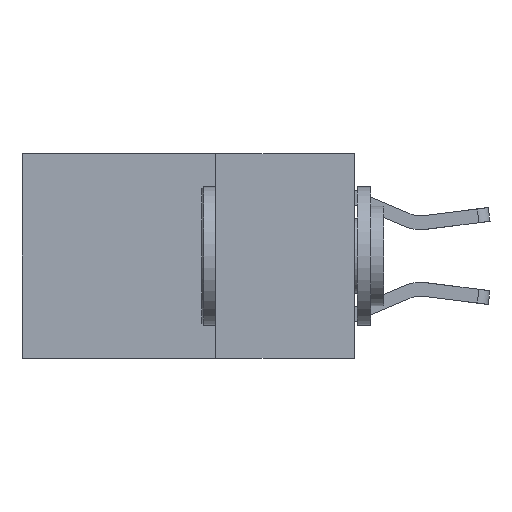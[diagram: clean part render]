
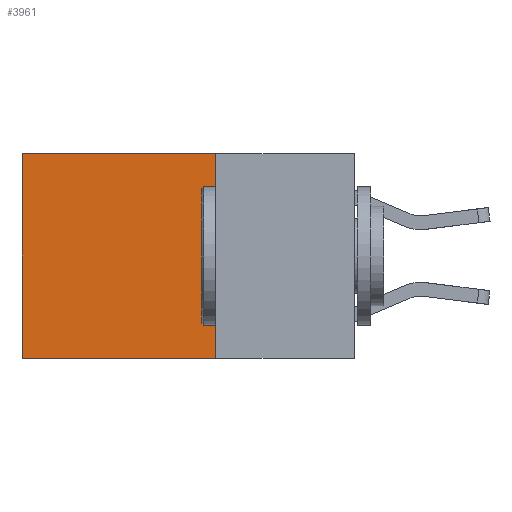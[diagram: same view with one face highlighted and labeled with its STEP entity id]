
A CAD part, left-side view. The second image highlights one B-rep face of the part: STEP entity #3961.
In plain terms, the highlighted planar face has unit normal (-1, 0, 0).
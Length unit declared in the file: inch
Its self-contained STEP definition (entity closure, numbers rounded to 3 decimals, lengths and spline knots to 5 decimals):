
#654 = DIRECTION ( 'NONE',  ( 1., 0., 0. ) ) ;
#752 = EDGE_LOOP ( 'NONE', ( #3261, #6210, #2704, #8444 ) ) ;
#809 = VECTOR ( 'NONE', #5398, 39.37008 ) ;
#868 = DIRECTION ( 'NONE',  ( 0., 0., -1. ) ) ;
#966 = CARTESIAN_POINT ( 'NONE',  ( 0.2625, 0.25, -0.37 ) ) ;
#1602 = LINE ( 'NONE', #6853, #809 ) ;
#1788 = CARTESIAN_POINT ( 'NONE',  ( 0.2625, 0.25, 0. ) ) ;
#2057 = VERTEX_POINT ( 'NONE', #5592 ) ;
#2075 = FACE_OUTER_BOUND ( 'NONE', #752, .T. ) ;
#2262 = DIRECTION ( 'NONE',  ( 0., 0., -1. ) ) ;
#2285 = LINE ( 'NONE', #6112, #8913 ) ;
#2596 = VECTOR ( 'NONE', #4803, 39.37008 ) ;
#2704 = ORIENTED_EDGE ( 'NONE', *, *, #4553, .F. ) ;
#2886 = VERTEX_POINT ( 'NONE', #6091 ) ;
#2995 = PLANE ( 'NONE',  #5045 ) ;
#3261 = ORIENTED_EDGE ( 'NONE', *, *, #8812, .T. ) ;
#3938 = VERTEX_POINT ( 'NONE', #8031 ) ;
#3961 = ADVANCED_FACE ( 'NONE', ( #2075 ), #2995, .F. ) ;
#4553 = EDGE_CURVE ( 'NONE', #2886, #2057, #1602, .T. ) ;
#4803 = DIRECTION ( 'NONE',  ( 0., 1., 0. ) ) ;
#5045 = AXIS2_PLACEMENT_3D ( 'NONE', #5085, #654, #2262 ) ;
#5085 = CARTESIAN_POINT ( 'NONE',  ( 0.2625, 0.25, 0. ) ) ;
#5398 = DIRECTION ( 'NONE',  ( 0., 0., -1. ) ) ;
#5475 = DIRECTION ( 'NONE',  ( 0., 1., 0. ) ) ;
#5592 = CARTESIAN_POINT ( 'NONE',  ( 0.2625, 0.25, -0.37 ) ) ;
#5602 = CARTESIAN_POINT ( 'NONE',  ( 0.2625, 0.6, -0.37 ) ) ;
#6091 = CARTESIAN_POINT ( 'NONE',  ( 0.2625, 0.25, 0. ) ) ;
#6112 = CARTESIAN_POINT ( 'NONE',  ( 0.2625, 0.6, 0. ) ) ;
#6170 = LINE ( 'NONE', #966, #6562 ) ;
#6210 = ORIENTED_EDGE ( 'NONE', *, *, #8962, .F. ) ;
#6375 = VERTEX_POINT ( 'NONE', #5602 ) ;
#6562 = VECTOR ( 'NONE', #5475, 39.37008 ) ;
#6853 = CARTESIAN_POINT ( 'NONE',  ( 0.2625, 0.25, 0. ) ) ;
#8031 = CARTESIAN_POINT ( 'NONE',  ( 0.2625, 0.6, 0. ) ) ;
#8444 = ORIENTED_EDGE ( 'NONE', *, *, #8603, .T. ) ;
#8603 = EDGE_CURVE ( 'NONE', #2886, #3938, #8651, .T. ) ;
#8651 = LINE ( 'NONE', #1788, #2596 ) ;
#8812 = EDGE_CURVE ( 'NONE', #3938, #6375, #2285, .T. ) ;
#8913 = VECTOR ( 'NONE', #868, 39.37008 ) ;
#8962 = EDGE_CURVE ( 'NONE', #2057, #6375, #6170, .T. ) ;
